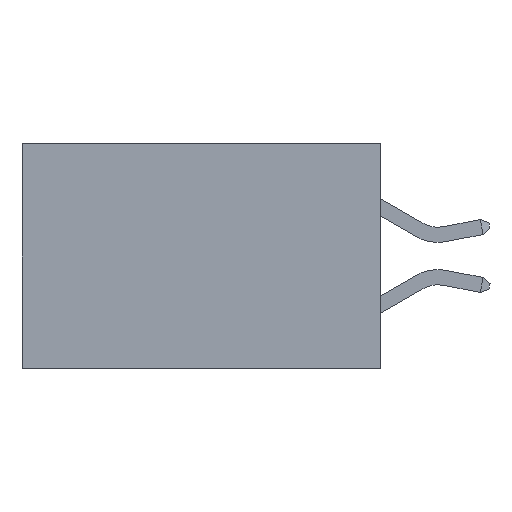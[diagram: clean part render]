
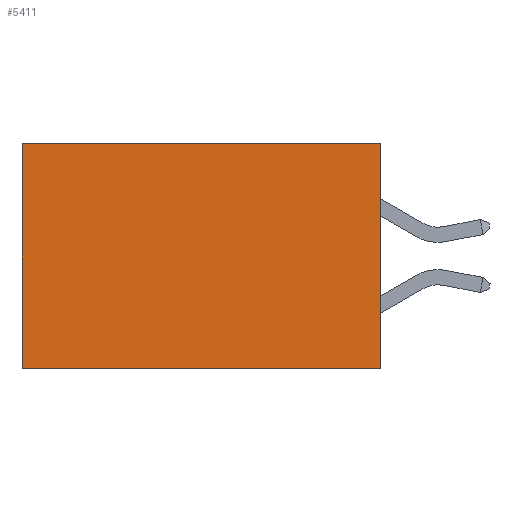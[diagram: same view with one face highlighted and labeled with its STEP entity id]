
A CAD part, left-side view. The second image highlights one B-rep face of the part: STEP entity #5411.
In plain terms, the highlighted planar face has unit normal (-1, 0, 0).
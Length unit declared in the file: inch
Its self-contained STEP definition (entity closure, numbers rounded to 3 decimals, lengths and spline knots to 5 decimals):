
#381 = VECTOR ( 'NONE', #7804, 39.37008 ) ;
#1272 = EDGE_LOOP ( 'NONE', ( #6140, #10087, #24349, #18004 ) ) ;
#2708 = LINE ( 'NONE', #10162, #8975 ) ;
#4298 = EDGE_CURVE ( 'NONE', #19015, #23092, #2708, .T. ) ;
#4571 = DIRECTION ( 'NONE',  ( 0., 1., 0. ) ) ;
#5284 = AXIS2_PLACEMENT_3D ( 'NONE', #15742, #14652, #14548 ) ;
#5411 = ADVANCED_FACE ( 'NONE', ( #8570 ), #15160, .F. ) ;
#5518 = EDGE_CURVE ( 'NONE', #19015, #18984, #5922, .T. ) ;
#5922 = LINE ( 'NONE', #7947, #381 ) ;
#6140 = ORIENTED_EDGE ( 'NONE', *, *, #17245, .T. ) ;
#7071 = CARTESIAN_POINT ( 'NONE',  ( 0.277, 0.59, 0. ) ) ;
#7804 = DIRECTION ( 'NONE',  ( 0., 1., 0. ) ) ;
#7947 = CARTESIAN_POINT ( 'NONE',  ( 0.277, 0., 0. ) ) ;
#8174 = DIRECTION ( 'NONE',  ( 0., 0., -1. ) ) ;
#8267 = VECTOR ( 'NONE', #8174, 39.37008 ) ;
#8570 = FACE_OUTER_BOUND ( 'NONE', #1272, .T. ) ;
#8754 = VERTEX_POINT ( 'NONE', #9234 ) ;
#8975 = VECTOR ( 'NONE', #10026, 39.37008 ) ;
#9234 = CARTESIAN_POINT ( 'NONE',  ( 0.277, 0.59, -0.37 ) ) ;
#10026 = DIRECTION ( 'NONE',  ( 0., 0., -1. ) ) ;
#10087 = ORIENTED_EDGE ( 'NONE', *, *, #17437, .F. ) ;
#10162 = CARTESIAN_POINT ( 'NONE',  ( 0.277, 0., -0.37 ) ) ;
#10226 = CARTESIAN_POINT ( 'NONE',  ( 0.277, 0.59, -0.37 ) ) ;
#12963 = CARTESIAN_POINT ( 'NONE',  ( 0.277, 0., -0.37 ) ) ;
#13878 = LINE ( 'NONE', #10226, #8267 ) ;
#14548 = DIRECTION ( 'NONE',  ( 0., 0., -1. ) ) ;
#14652 = DIRECTION ( 'NONE',  ( 1., 0., 0. ) ) ;
#15160 = PLANE ( 'NONE',  #5284 ) ;
#15742 = CARTESIAN_POINT ( 'NONE',  ( 0.277, 0., -0.37 ) ) ;
#17245 = EDGE_CURVE ( 'NONE', #18984, #8754, #13878, .T. ) ;
#17437 = EDGE_CURVE ( 'NONE', #23092, #8754, #25778, .T. ) ;
#18004 = ORIENTED_EDGE ( 'NONE', *, *, #5518, .T. ) ;
#18984 = VERTEX_POINT ( 'NONE', #7071 ) ;
#19015 = VERTEX_POINT ( 'NONE', #19643 ) ;
#19643 = CARTESIAN_POINT ( 'NONE',  ( 0.277, 0., 0. ) ) ;
#19650 = VECTOR ( 'NONE', #4571, 39.37008 ) ;
#20270 = CARTESIAN_POINT ( 'NONE',  ( 0.277, 0., -0.37 ) ) ;
#23092 = VERTEX_POINT ( 'NONE', #20270 ) ;
#24349 = ORIENTED_EDGE ( 'NONE', *, *, #4298, .F. ) ;
#25778 = LINE ( 'NONE', #12963, #19650 ) ;
